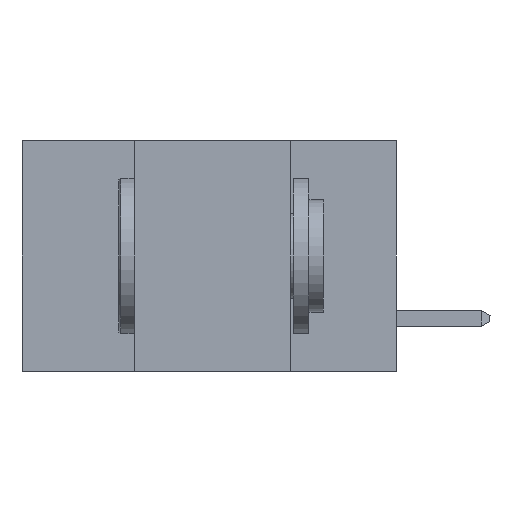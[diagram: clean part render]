
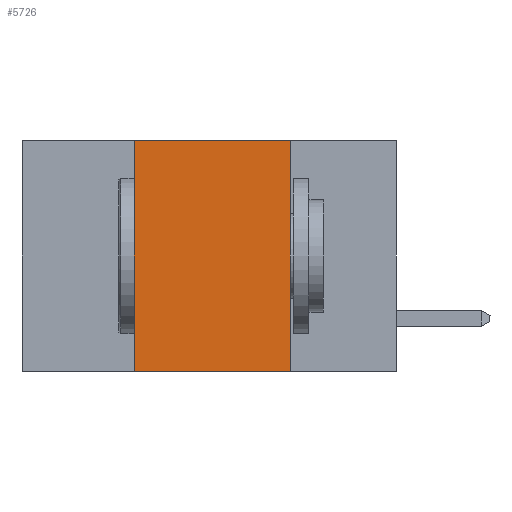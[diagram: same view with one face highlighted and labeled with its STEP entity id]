
A CAD part, left-side view. The second image highlights one B-rep face of the part: STEP entity #5726.
In plain terms, the highlighted planar face has unit normal (-1, 0, 0).
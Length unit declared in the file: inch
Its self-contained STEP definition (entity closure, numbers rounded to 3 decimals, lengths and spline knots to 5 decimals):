
#126 = CARTESIAN_POINT ( 'NONE',  ( 0., 0.42, 0. ) ) ;
#311 = VECTOR ( 'NONE', #11742, 39.37008 ) ;
#652 = VERTEX_POINT ( 'NONE', #20295 ) ;
#670 = EDGE_CURVE ( 'NONE', #652, #20653, #1857, .T. ) ;
#1857 = LINE ( 'NONE', #10418, #8748 ) ;
#2444 = DIRECTION ( 'NONE',  ( 0., -1., 0. ) ) ;
#3037 = DIRECTION ( 'NONE',  ( 1., 0., 0. ) ) ;
#3125 = CARTESIAN_POINT ( 'NONE',  ( 0., 0.17, -0.37 ) ) ;
#4247 = VERTEX_POINT ( 'NONE', #3125 ) ;
#5056 = VECTOR ( 'NONE', #17762, 39.37008 ) ;
#5141 = EDGE_CURVE ( 'NONE', #5480, #652, #9389, .T. ) ;
#5480 = VERTEX_POINT ( 'NONE', #9212 ) ;
#5725 = VECTOR ( 'NONE', #8886, 39.37008 ) ;
#5726 = ADVANCED_FACE ( 'NONE', ( #13408 ), #9597, .F. ) ;
#6241 = DIRECTION ( 'NONE',  ( 0., 0., -1. ) ) ;
#7394 = ORIENTED_EDGE ( 'NONE', *, *, #19794, .F. ) ;
#8748 = VECTOR ( 'NONE', #2444, 39.37008 ) ;
#8886 = DIRECTION ( 'NONE',  ( 0., 0., -1. ) ) ;
#9212 = CARTESIAN_POINT ( 'NONE',  ( 0., 0.42, -0.37 ) ) ;
#9286 = EDGE_CURVE ( 'NONE', #5480, #4247, #13775, .T. ) ;
#9389 = LINE ( 'NONE', #126, #5056 ) ;
#9597 = PLANE ( 'NONE',  #17329 ) ;
#10418 = CARTESIAN_POINT ( 'NONE',  ( 0., 0.6, 0. ) ) ;
#10928 = ORIENTED_EDGE ( 'NONE', *, *, #5141, .F. ) ;
#11742 = DIRECTION ( 'NONE',  ( 0., -1., 0. ) ) ;
#13408 = FACE_OUTER_BOUND ( 'NONE', #19634, .T. ) ;
#13775 = LINE ( 'NONE', #16718, #311 ) ;
#14849 = LINE ( 'NONE', #18690, #5725 ) ;
#16017 = CARTESIAN_POINT ( 'NONE',  ( 0., 0.6, 0. ) ) ;
#16718 = CARTESIAN_POINT ( 'NONE',  ( 0., 0.6, -0.37 ) ) ;
#17329 = AXIS2_PLACEMENT_3D ( 'NONE', #16017, #3037, #6241 ) ;
#17762 = DIRECTION ( 'NONE',  ( 0., 0., 1. ) ) ;
#18690 = CARTESIAN_POINT ( 'NONE',  ( 0., 0.17, 0. ) ) ;
#18830 = ORIENTED_EDGE ( 'NONE', *, *, #670, .F. ) ;
#19631 = CARTESIAN_POINT ( 'NONE',  ( 0., 0.17, 0. ) ) ;
#19634 = EDGE_LOOP ( 'NONE', ( #7394, #18830, #10928, #20025 ) ) ;
#19794 = EDGE_CURVE ( 'NONE', #20653, #4247, #14849, .T. ) ;
#20025 = ORIENTED_EDGE ( 'NONE', *, *, #9286, .T. ) ;
#20295 = CARTESIAN_POINT ( 'NONE',  ( 0., 0.42, 0. ) ) ;
#20653 = VERTEX_POINT ( 'NONE', #19631 ) ;
